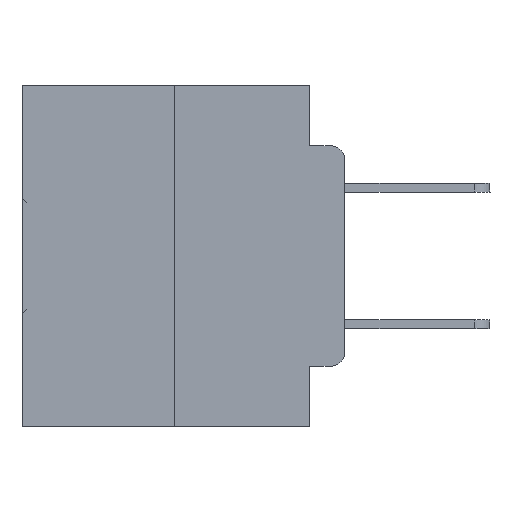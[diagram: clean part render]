
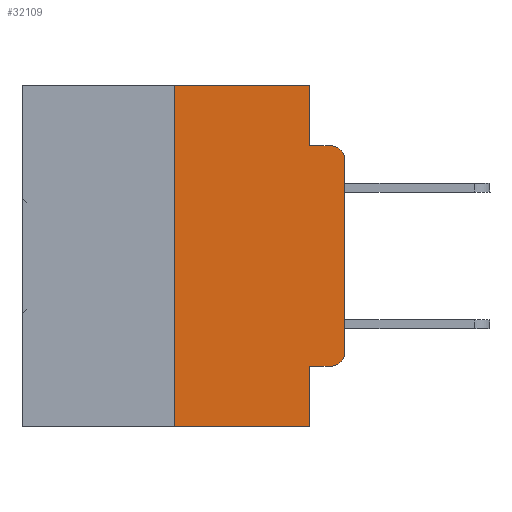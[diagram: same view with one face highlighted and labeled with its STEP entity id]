
A CAD part, left-side view. The second image highlights one B-rep face of the part: STEP entity #32109.
In plain terms, the highlighted planar face has unit normal (-1, 0, 0).
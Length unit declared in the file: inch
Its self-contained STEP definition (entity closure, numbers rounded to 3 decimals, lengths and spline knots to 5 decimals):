
#153 = VECTOR ( 'NONE', #23600, 39.37008 ) ;
#1321 = ORIENTED_EDGE ( 'NONE', *, *, #8702, .F. ) ;
#2056 = VECTOR ( 'NONE', #20355, 39.37008 ) ;
#2367 = VERTEX_POINT ( 'NONE', #27745 ) ;
#2464 = CARTESIAN_POINT ( 'NONE',  ( 0., 0., -0.3915 ) ) ;
#2973 = EDGE_CURVE ( 'NONE', #22318, #16037, #25742, .T. ) ;
#3193 = CARTESIAN_POINT ( 'NONE',  ( 0., 0.25, 0. ) ) ;
#4973 = CARTESIAN_POINT ( 'NONE',  ( 0., 0.02, -0.4115 ) ) ;
#5573 = DIRECTION ( 'NONE',  ( 0., 0., -1. ) ) ;
#5575 = DIRECTION ( 'NONE',  ( 0., -1., 0. ) ) ;
#6107 = LINE ( 'NONE', #23961, #25101 ) ;
#6646 = VERTEX_POINT ( 'NONE', #26377 ) ;
#6713 = ORIENTED_EDGE ( 'NONE', *, *, #26518, .T. ) ;
#6754 = VERTEX_POINT ( 'NONE', #22065 ) ;
#7459 = CARTESIAN_POINT ( 'NONE',  ( 0., 0., -0.1085 ) ) ;
#7460 = CARTESIAN_POINT ( 'NONE',  ( 0., 0.02, -0.3915 ) ) ;
#7600 = VECTOR ( 'NONE', #8792, 39.37008 ) ;
#7664 = VERTEX_POINT ( 'NONE', #24762 ) ;
#7695 = ORIENTED_EDGE ( 'NONE', *, *, #2973, .T. ) ;
#7960 = CARTESIAN_POINT ( 'NONE',  ( 0., 0., 0. ) ) ;
#8218 = LINE ( 'NONE', #7960, #153 ) ;
#8660 = EDGE_CURVE ( 'NONE', #20158, #13757, #25464, .T. ) ;
#8702 = EDGE_CURVE ( 'NONE', #31141, #6754, #18614, .T. ) ;
#8743 = FACE_OUTER_BOUND ( 'NONE', #32438, .T. ) ;
#8792 = DIRECTION ( 'NONE',  ( 0., 0., 1. ) ) ;
#8885 = LINE ( 'NONE', #23084, #2056 ) ;
#9906 = AXIS2_PLACEMENT_3D ( 'NONE', #29878, #14679, #14569 ) ;
#10326 = LINE ( 'NONE', #16067, #32658 ) ;
#10565 = CARTESIAN_POINT ( 'NONE',  ( 0., 0.25, -0.5 ) ) ;
#10834 = ORIENTED_EDGE ( 'NONE', *, *, #32275, .T. ) ;
#11164 = PLANE ( 'NONE',  #13375 ) ;
#11334 = VECTOR ( 'NONE', #5575, 39.37008 ) ;
#11498 = DIRECTION ( 'NONE',  ( 1., 0., 0. ) ) ;
#11641 = VECTOR ( 'NONE', #22158, 39.37008 ) ;
#13375 = AXIS2_PLACEMENT_3D ( 'NONE', #26613, #11498, #27054 ) ;
#13757 = VERTEX_POINT ( 'NONE', #3193 ) ;
#14054 = ORIENTED_EDGE ( 'NONE', *, *, #17725, .F. ) ;
#14569 = DIRECTION ( 'NONE',  ( 0., 0., -1. ) ) ;
#14679 = DIRECTION ( 'NONE',  ( -1., 0., 0. ) ) ;
#15722 = DIRECTION ( 'NONE',  ( -1., 0., 0. ) ) ;
#16037 = VERTEX_POINT ( 'NONE', #2464 ) ;
#16067 = CARTESIAN_POINT ( 'NONE',  ( 0., 0.051, 0. ) ) ;
#16608 = CARTESIAN_POINT ( 'NONE',  ( 0., 0.051, 0. ) ) ;
#16612 = VERTEX_POINT ( 'NONE', #7459 ) ;
#17725 = EDGE_CURVE ( 'NONE', #13757, #31141, #6107, .T. ) ;
#18614 = LINE ( 'NONE', #16608, #11641 ) ;
#19099 = LINE ( 'NONE', #21289, #11334 ) ;
#19364 = DIRECTION ( 'NONE',  ( 0., 0., -1. ) ) ;
#19715 = EDGE_CURVE ( 'NONE', #2367, #7664, #10326, .T. ) ;
#19812 = CARTESIAN_POINT ( 'NONE',  ( 0., 0.051, -0.0885 ) ) ;
#20107 = ORIENTED_EDGE ( 'NONE', *, *, #28164, .F. ) ;
#20158 = VERTEX_POINT ( 'NONE', #10565 ) ;
#20355 = DIRECTION ( 'NONE',  ( 0., -1., 0. ) ) ;
#20364 = LINE ( 'NONE', #19812, #28468 ) ;
#21289 = CARTESIAN_POINT ( 'NONE',  ( 0., 0.051, -0.4115 ) ) ;
#21473 = ORIENTED_EDGE ( 'NONE', *, *, #8660, .F. ) ;
#21582 = DIRECTION ( 'NONE',  ( 0., -1., 0. ) ) ;
#22023 = EDGE_CURVE ( 'NONE', #20158, #7664, #8885, .T. ) ;
#22065 = CARTESIAN_POINT ( 'NONE',  ( 0., 0.051, -0.0885 ) ) ;
#22158 = DIRECTION ( 'NONE',  ( 0., 0., -1. ) ) ;
#22318 = VERTEX_POINT ( 'NONE', #4973 ) ;
#22920 = CIRCLE ( 'NONE', #9906, 0.02 ) ;
#23084 = CARTESIAN_POINT ( 'NONE',  ( 0., 0.473, -0.5 ) ) ;
#23600 = DIRECTION ( 'NONE',  ( 0., 0., 1. ) ) ;
#23961 = CARTESIAN_POINT ( 'NONE',  ( 0., 0.473, 0. ) ) ;
#24327 = CARTESIAN_POINT ( 'NONE',  ( 0., 0.25, 0. ) ) ;
#24762 = CARTESIAN_POINT ( 'NONE',  ( 0., 0.051, -0.5 ) ) ;
#25101 = VECTOR ( 'NONE', #21582, 39.37008 ) ;
#25464 = LINE ( 'NONE', #24327, #7600 ) ;
#25727 = EDGE_CURVE ( 'NONE', #16037, #16612, #8218, .T. ) ;
#25742 = CIRCLE ( 'NONE', #33010, 0.02 ) ;
#26377 = CARTESIAN_POINT ( 'NONE',  ( 0., 0.02, -0.0885 ) ) ;
#26518 = EDGE_CURVE ( 'NONE', #2367, #22318, #19099, .T. ) ;
#26613 = CARTESIAN_POINT ( 'NONE',  ( 0., 0.473, 0. ) ) ;
#27054 = DIRECTION ( 'NONE',  ( 0., 0., -1. ) ) ;
#27745 = CARTESIAN_POINT ( 'NONE',  ( 0., 0.051, -0.4115 ) ) ;
#28164 = EDGE_CURVE ( 'NONE', #6754, #6646, #20364, .T. ) ;
#28468 = VECTOR ( 'NONE', #33187, 39.37008 ) ;
#28806 = ORIENTED_EDGE ( 'NONE', *, *, #25727, .T. ) ;
#29806 = ORIENTED_EDGE ( 'NONE', *, *, #22023, .T. ) ;
#29878 = CARTESIAN_POINT ( 'NONE',  ( 0., 0.02, -0.1085 ) ) ;
#31141 = VERTEX_POINT ( 'NONE', #33234 ) ;
#32109 = ADVANCED_FACE ( 'NONE', ( #8743 ), #11164, .F. ) ;
#32275 = EDGE_CURVE ( 'NONE', #16612, #6646, #22920, .T. ) ;
#32438 = EDGE_LOOP ( 'NONE', ( #28806, #10834, #20107, #1321, #14054, #21473, #29806, #32486, #6713, #7695 ) ) ;
#32486 = ORIENTED_EDGE ( 'NONE', *, *, #19715, .F. ) ;
#32658 = VECTOR ( 'NONE', #19364, 39.37008 ) ;
#33010 = AXIS2_PLACEMENT_3D ( 'NONE', #7460, #15722, #5573 ) ;
#33187 = DIRECTION ( 'NONE',  ( 0., -1., 0. ) ) ;
#33234 = CARTESIAN_POINT ( 'NONE',  ( 0., 0.051, 0. ) ) ;
